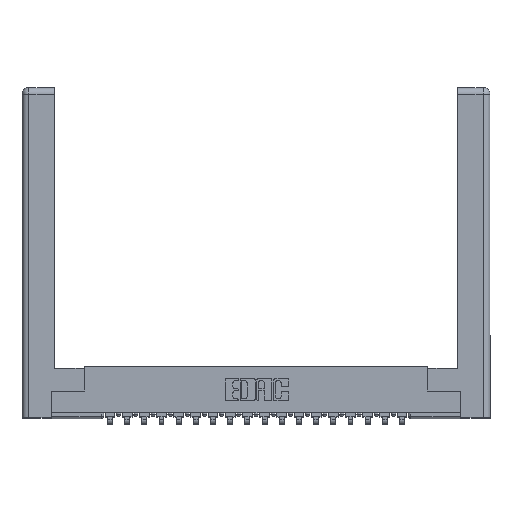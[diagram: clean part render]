
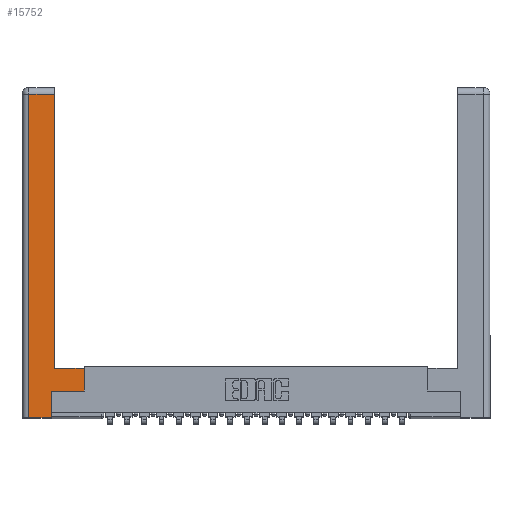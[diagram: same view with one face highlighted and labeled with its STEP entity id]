
A CAD part, top view. The second image highlights one B-rep face of the part: STEP entity #15752.
In plain terms, the highlighted planar face has unit normal (0, 0, 1).
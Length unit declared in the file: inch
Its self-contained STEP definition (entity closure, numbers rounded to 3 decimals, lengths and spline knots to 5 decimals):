
#554 = CARTESIAN_POINT ( 'NONE',  ( 0.295, 2.94, 0. ) ) ;
#569 = DIRECTION ( 'NONE',  ( -1., 0., 0. ) ) ;
#669 = EDGE_CURVE ( 'NONE', #5821, #21684, #16749, .T. ) ;
#953 = VECTOR ( 'NONE', #13633, 39.37008 ) ;
#1183 = CARTESIAN_POINT ( 'NONE',  ( 0.265, 0.245, 0. ) ) ;
#1212 = DIRECTION ( 'NONE',  ( 0., -1., 0. ) ) ;
#1327 = EDGE_CURVE ( 'NONE', #10755, #7370, #8215, .T. ) ;
#1634 = CARTESIAN_POINT ( 'NONE',  ( 0.0615, 0., 0. ) ) ;
#1757 = EDGE_CURVE ( 'NONE', #9813, #5821, #10616, .T. ) ;
#2221 = CARTESIAN_POINT ( 'NONE',  ( 0.295, 0.45, 0. ) ) ;
#2483 = VECTOR ( 'NONE', #20182, 39.37008 ) ;
#2830 = ORIENTED_EDGE ( 'NONE', *, *, #10002, .T. ) ;
#3052 = LINE ( 'NONE', #3786, #16248 ) ;
#3546 = DIRECTION ( 'NONE',  ( 0., 1., 0. ) ) ;
#3786 = CARTESIAN_POINT ( 'NONE',  ( 0.265, 0.245, 0. ) ) ;
#3916 = LINE ( 'NONE', #9125, #9437 ) ;
#5175 = CARTESIAN_POINT ( 'NONE',  ( 0.295, 0.45, 0. ) ) ;
#5533 = DIRECTION ( 'NONE',  ( 0., 1., 0. ) ) ;
#5821 = VERTEX_POINT ( 'NONE', #5175 ) ;
#6237 = CARTESIAN_POINT ( 'NONE',  ( 0., 0., 0. ) ) ;
#7370 = VERTEX_POINT ( 'NONE', #1634 ) ;
#8215 = LINE ( 'NONE', #10934, #18557 ) ;
#8359 = CARTESIAN_POINT ( 'NONE',  ( 0.0615, 2.94, 0. ) ) ;
#8500 = ORIENTED_EDGE ( 'NONE', *, *, #15021, .T. ) ;
#9009 = ORIENTED_EDGE ( 'NONE', *, *, #21388, .T. ) ;
#9067 = VERTEX_POINT ( 'NONE', #13397 ) ;
#9125 = CARTESIAN_POINT ( 'NONE',  ( 0.565, 0.245, 0. ) ) ;
#9195 = ORIENTED_EDGE ( 'NONE', *, *, #1327, .T. ) ;
#9437 = VECTOR ( 'NONE', #16098, 39.37008 ) ;
#9813 = VERTEX_POINT ( 'NONE', #10399 ) ;
#10002 = EDGE_CURVE ( 'NONE', #11169, #9067, #3916, .T. ) ;
#10078 = CARTESIAN_POINT ( 'NONE',  ( 0.265, 0., 0. ) ) ;
#10325 = ORIENTED_EDGE ( 'NONE', *, *, #669, .T. ) ;
#10399 = CARTESIAN_POINT ( 'NONE',  ( 0.565, 0.45, 0. ) ) ;
#10448 = VERTEX_POINT ( 'NONE', #17405 ) ;
#10616 = LINE ( 'NONE', #2221, #19600 ) ;
#10755 = VERTEX_POINT ( 'NONE', #12965 ) ;
#10934 = CARTESIAN_POINT ( 'NONE',  ( 0.0615, 0., 0. ) ) ;
#11169 = VERTEX_POINT ( 'NONE', #1183 ) ;
#11183 = DIRECTION ( 'NONE',  ( 0., 0., -1. ) ) ;
#11919 = CARTESIAN_POINT ( 'NONE',  ( 0.565, 0.45, 0. ) ) ;
#12111 = ORIENTED_EDGE ( 'NONE', *, *, #1757, .T. ) ;
#12292 = VECTOR ( 'NONE', #3546, 39.37008 ) ;
#12760 = PLANE ( 'NONE',  #18095 ) ;
#12965 = CARTESIAN_POINT ( 'NONE',  ( 0.0615, 2.94, 0. ) ) ;
#13154 = ORIENTED_EDGE ( 'NONE', *, *, #19764, .T. ) ;
#13397 = CARTESIAN_POINT ( 'NONE',  ( 0.565, 0.245, 0. ) ) ;
#13633 = DIRECTION ( 'NONE',  ( 1., 0., 0. ) ) ;
#13779 = EDGE_LOOP ( 'NONE', ( #10325, #9009, #9195, #19956, #8500, #2830, #13154, #12111 ) ) ;
#14533 = DIRECTION ( 'NONE',  ( -1., 0., 0. ) ) ;
#14634 = VECTOR ( 'NONE', #17153, 39.37008 ) ;
#15021 = EDGE_CURVE ( 'NONE', #10448, #11169, #3052, .T. ) ;
#15752 = ADVANCED_FACE ( 'NONE', ( #20440 ), #12760, .F. ) ;
#15938 = LINE ( 'NONE', #8359, #2483 ) ;
#16098 = DIRECTION ( 'NONE',  ( 1., 0., 0. ) ) ;
#16248 = VECTOR ( 'NONE', #5533, 39.37008 ) ;
#16749 = LINE ( 'NONE', #18670, #14634 ) ;
#17153 = DIRECTION ( 'NONE',  ( 0., 1., 0. ) ) ;
#17334 = LINE ( 'NONE', #11919, #12292 ) ;
#17405 = CARTESIAN_POINT ( 'NONE',  ( 0.265, 0., 0. ) ) ;
#18095 = AXIS2_PLACEMENT_3D ( 'NONE', #6237, #11183, #14533 ) ;
#18557 = VECTOR ( 'NONE', #1212, 39.37008 ) ;
#18670 = CARTESIAN_POINT ( 'NONE',  ( 0.295, 3., 0. ) ) ;
#18904 = LINE ( 'NONE', #10078, #953 ) ;
#19600 = VECTOR ( 'NONE', #569, 39.37008 ) ;
#19764 = EDGE_CURVE ( 'NONE', #9067, #9813, #17334, .T. ) ;
#19788 = EDGE_CURVE ( 'NONE', #7370, #10448, #18904, .T. ) ;
#19956 = ORIENTED_EDGE ( 'NONE', *, *, #19788, .T. ) ;
#20182 = DIRECTION ( 'NONE',  ( -1., 0., 0. ) ) ;
#20440 = FACE_OUTER_BOUND ( 'NONE', #13779, .T. ) ;
#21388 = EDGE_CURVE ( 'NONE', #21684, #10755, #15938, .T. ) ;
#21684 = VERTEX_POINT ( 'NONE', #554 ) ;
